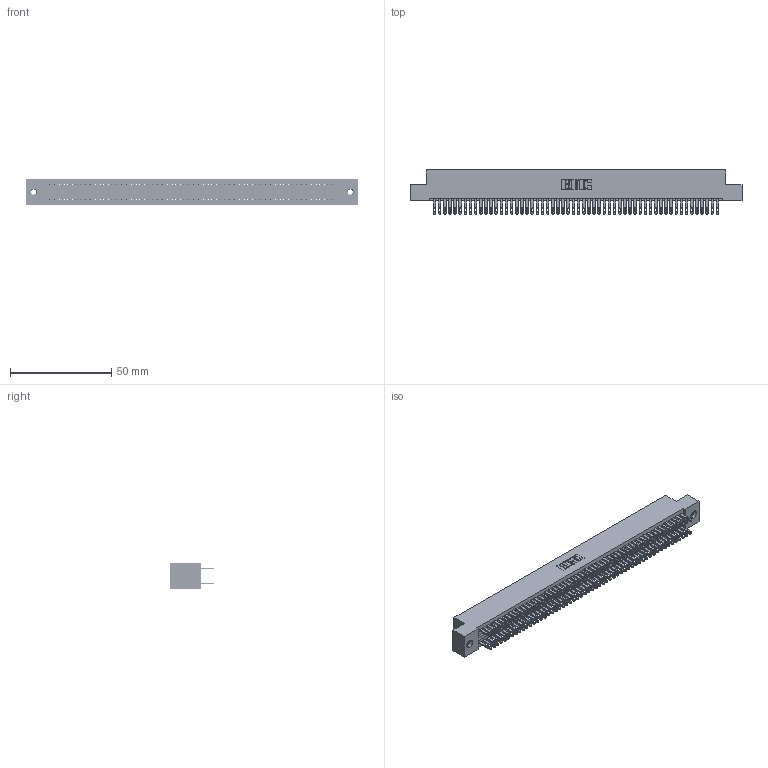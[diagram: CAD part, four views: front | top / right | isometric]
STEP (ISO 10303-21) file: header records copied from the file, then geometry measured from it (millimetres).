
FILE_DESCRIPTION (( 'STEP AP203' ), '1' );
FILE_NAME ('325-112-500-207.STEP', '2020-02-25T07:47:45', ( '' ), ( '' ), 'SwSTEP 2.0', 'SolidWorks 2016', '' );
FILE_SCHEMA (( 'CONFIG_CONTROL_DESIGN' ));
Length unit declared in the file: inch
Products named in the file (4): 325-112-500-207; 325-292-001_325-293-100; 325 Part_TI; 345-250-001_345-250-005-103
Assembly tree (115 placements, depth 2):
  325-112-500-207
    325 Part_TI
    325-292-001_325-293-100  x112
    345-250-001_345-250-005-103  x2
Bounding box: 163.96 x 21.84 x 12.45 mm (x, y, z)
Volume: 21620.5 mm3; surface area: 27698.1 mm2
Topology: 115 solids, 115 shells, 5550 faces, 16911 edges, 11266 vertices
Faces by surface type: plane 3462, cylinder 2072, cone 12, torus 4
Entity records: 35332 total; most frequent: CARTESIAN_POINT 5821, ORIENTED_EDGE 5750, DIRECTION 4981, EDGE_CURVE 2875, LINE 2723, VECTOR 2723, VERTEX_POINT 1912, AXIS2_PLACEMENT_3D 1129
